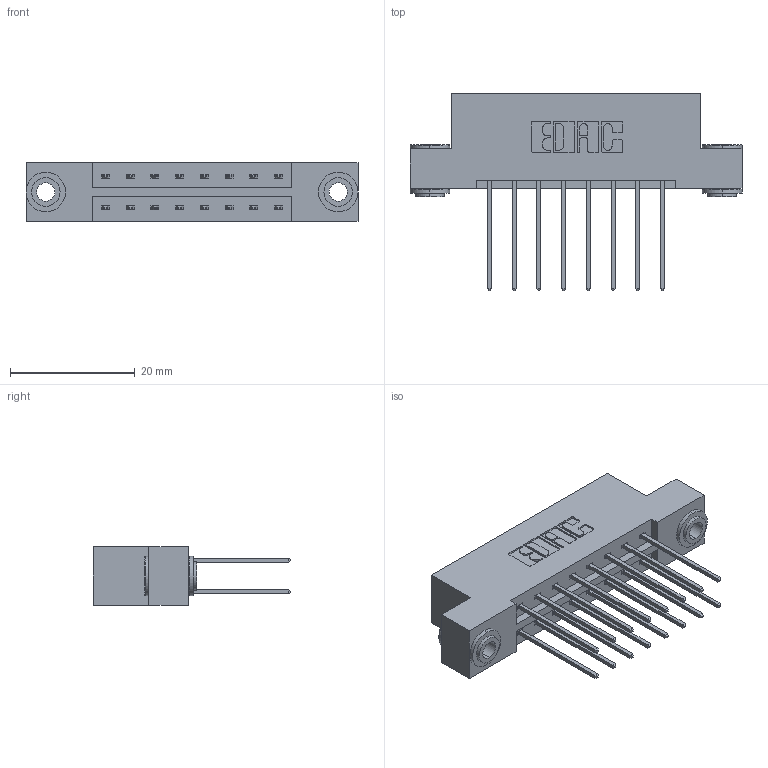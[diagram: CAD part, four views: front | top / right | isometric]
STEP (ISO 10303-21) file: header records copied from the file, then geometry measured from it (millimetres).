
FILE_DESCRIPTION (( 'STEP AP203' ), '1' );
FILE_NAME ('833-016-542-203.STEP', '2020-05-31T18:13:34', ( '' ), ( '' ), 'SwSTEP 2.0', 'SolidWorks 2020', '' );
FILE_SCHEMA (( 'CONFIG_CONTROL_DESIGN' ));
Length unit declared in the file: inch
Products named in the file (4): 345-250-002_345-250-002-102; 833 Part_Flush - .156 Dia - TH; 345-292-001_345-293-142; 833-016-542-203
Assembly tree (19 placements, depth 2):
  833-016-542-203
    833 Part_Flush - .156 Dia - TH
    345-292-001_345-293-142  x16
    345-250-002_345-250-002-102  x2
Bounding box: 53.24 x 31.63 x 9.4 mm (x, y, z)
Volume: 5211.4 mm3; surface area: 6385.7 mm2
Topology: 19 solids, 19 shells, 984 faces, 2867 edges, 1886 vertices
Faces by surface type: plane 656, cylinder 320, cone 8
Entity records: 10212 total; most frequent: CARTESIAN_POINT 1709, ORIENTED_EDGE 1638, DIRECTION 1553, EDGE_CURVE 819, VECTOR 667, LINE 667, VERTEX_POINT 542, AXIS2_PLACEMENT_3D 443
